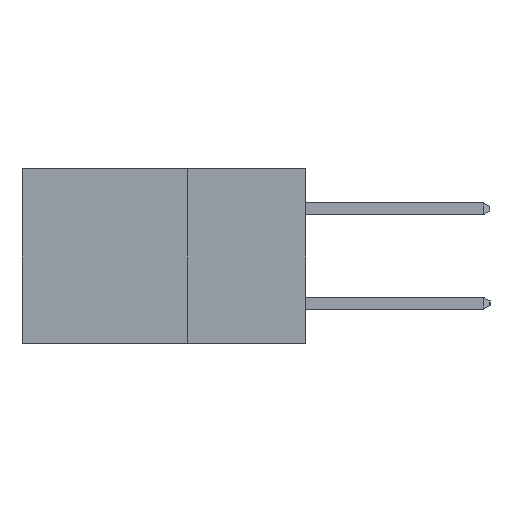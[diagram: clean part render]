
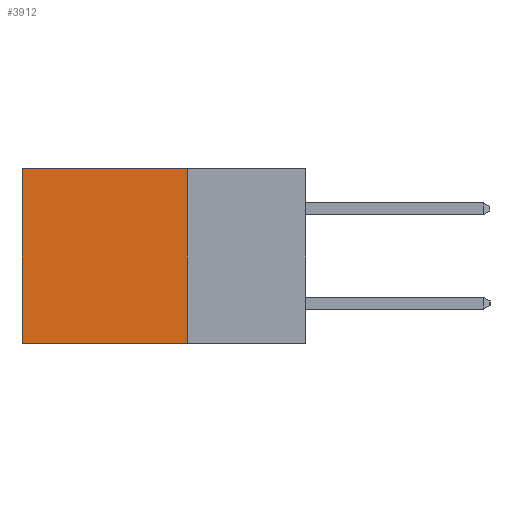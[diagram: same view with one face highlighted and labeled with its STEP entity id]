
A CAD part, left-side view. The second image highlights one B-rep face of the part: STEP entity #3912.
In plain terms, the highlighted planar face has unit normal (-1, 0, 0).
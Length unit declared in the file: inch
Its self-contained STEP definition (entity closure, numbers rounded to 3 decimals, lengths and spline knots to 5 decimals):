
#59 = DIRECTION ( 'NONE',  ( 0., 1., 0. ) ) ;
#589 = ORIENTED_EDGE ( 'NONE', *, *, #6302, .T. ) ;
#751 = FACE_OUTER_BOUND ( 'NONE', #4554, .T. ) ;
#853 = CARTESIAN_POINT ( 'NONE',  ( 0.2615, 0.25, -0.37 ) ) ;
#2718 = EDGE_CURVE ( 'NONE', #17151, #10188, #5696, .T. ) ;
#3912 = ADVANCED_FACE ( 'NONE', ( #751 ), #10006, .F. ) ;
#4398 = CARTESIAN_POINT ( 'NONE',  ( 0.2615, 0.25, 0. ) ) ;
#4554 = EDGE_LOOP ( 'NONE', ( #12636, #16957, #6162, #589 ) ) ;
#4942 = EDGE_CURVE ( 'NONE', #15570, #15535, #16880, .T. ) ;
#5092 = VECTOR ( 'NONE', #12371, 39.37008 ) ;
#5696 = LINE ( 'NONE', #13972, #13904 ) ;
#5773 = CARTESIAN_POINT ( 'NONE',  ( 0.2615, 0.6, -0.37 ) ) ;
#5991 = EDGE_CURVE ( 'NONE', #10188, #15535, #18474, .T. ) ;
#6162 = ORIENTED_EDGE ( 'NONE', *, *, #2718, .F. ) ;
#6302 = EDGE_CURVE ( 'NONE', #17151, #15570, #9229, .T. ) ;
#8364 = CARTESIAN_POINT ( 'NONE',  ( 0.2615, 0.25, -0.37 ) ) ;
#9229 = LINE ( 'NONE', #12904, #5092 ) ;
#9878 = DIRECTION ( 'NONE',  ( 0., 0., -1. ) ) ;
#9925 = DIRECTION ( 'NONE',  ( 1., 0., 0. ) ) ;
#9947 = CARTESIAN_POINT ( 'NONE',  ( 0.2615, 0.25, -0.37 ) ) ;
#10006 = PLANE ( 'NONE',  #16162 ) ;
#10188 = VERTEX_POINT ( 'NONE', #8364 ) ;
#12371 = DIRECTION ( 'NONE',  ( 0., 1., 0. ) ) ;
#12542 = CARTESIAN_POINT ( 'NONE',  ( 0.2615, 0.6, -0.37 ) ) ;
#12636 = ORIENTED_EDGE ( 'NONE', *, *, #4942, .T. ) ;
#12870 = VECTOR ( 'NONE', #15317, 39.37008 ) ;
#12904 = CARTESIAN_POINT ( 'NONE',  ( 0.2615, 0.25, 0. ) ) ;
#13904 = VECTOR ( 'NONE', #14234, 39.37008 ) ;
#13972 = CARTESIAN_POINT ( 'NONE',  ( 0.2615, 0.25, -0.37 ) ) ;
#14019 = VECTOR ( 'NONE', #59, 39.37008 ) ;
#14234 = DIRECTION ( 'NONE',  ( 0., 0., -1. ) ) ;
#15317 = DIRECTION ( 'NONE',  ( 0., 0., -1. ) ) ;
#15535 = VERTEX_POINT ( 'NONE', #5773 ) ;
#15570 = VERTEX_POINT ( 'NONE', #19507 ) ;
#16162 = AXIS2_PLACEMENT_3D ( 'NONE', #9947, #9925, #9878 ) ;
#16880 = LINE ( 'NONE', #12542, #12870 ) ;
#16957 = ORIENTED_EDGE ( 'NONE', *, *, #5991, .F. ) ;
#17151 = VERTEX_POINT ( 'NONE', #4398 ) ;
#18474 = LINE ( 'NONE', #853, #14019 ) ;
#19507 = CARTESIAN_POINT ( 'NONE',  ( 0.2615, 0.6, 0. ) ) ;
